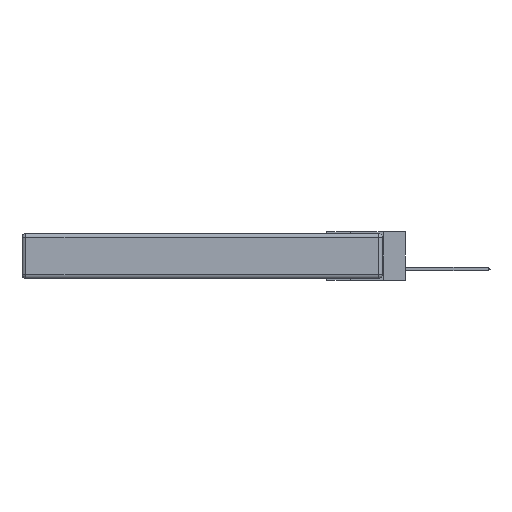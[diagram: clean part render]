
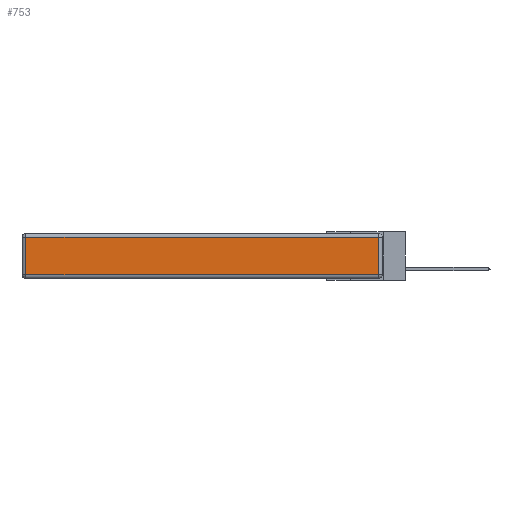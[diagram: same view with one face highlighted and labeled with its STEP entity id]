
A CAD part, left-side view. The second image highlights one B-rep face of the part: STEP entity #753.
In plain terms, the highlighted planar face has unit normal (-1, 0, 0).
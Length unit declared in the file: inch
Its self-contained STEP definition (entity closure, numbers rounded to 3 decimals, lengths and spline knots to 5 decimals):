
#368 = EDGE_LOOP ( 'NONE', ( #6612, #5423, #10526, #2184 ) ) ;
#753 = ADVANCED_FACE ( 'NONE', ( #3915 ), #14682, .T. ) ;
#966 = VERTEX_POINT ( 'NONE', #8173 ) ;
#1011 = VERTEX_POINT ( 'NONE', #5994 ) ;
#1536 = LINE ( 'NONE', #10041, #2439 ) ;
#1815 = DIRECTION ( 'NONE',  ( 0., 1., 0. ) ) ;
#1923 = CARTESIAN_POINT ( 'NONE',  ( 0., 0., -0.343 ) ) ;
#2184 = ORIENTED_EDGE ( 'NONE', *, *, #7579, .T. ) ;
#2439 = VECTOR ( 'NONE', #11105, 39.37008 ) ;
#2649 = AXIS2_PLACEMENT_3D ( 'NONE', #1923, #10116, #7851 ) ;
#3911 = LINE ( 'NONE', #10611, #14487 ) ;
#3915 = FACE_OUTER_BOUND ( 'NONE', #368, .T. ) ;
#4009 = VERTEX_POINT ( 'NONE', #6606 ) ;
#4756 = VERTEX_POINT ( 'NONE', #5354 ) ;
#5354 = CARTESIAN_POINT ( 'NONE',  ( 0., 2.72, -0.313 ) ) ;
#5423 = ORIENTED_EDGE ( 'NONE', *, *, #12907, .T. ) ;
#5526 = CARTESIAN_POINT ( 'NONE',  ( 0., 2.75, -0.03 ) ) ;
#5942 = VECTOR ( 'NONE', #14216, 39.37008 ) ;
#5994 = CARTESIAN_POINT ( 'NONE',  ( 0., 2.72, -0.03 ) ) ;
#6606 = CARTESIAN_POINT ( 'NONE',  ( 0., 0.03, -0.313 ) ) ;
#6612 = ORIENTED_EDGE ( 'NONE', *, *, #12683, .T. ) ;
#7579 = EDGE_CURVE ( 'NONE', #1011, #4756, #9051, .T. ) ;
#7851 = DIRECTION ( 'NONE',  ( 0., 0., 1. ) ) ;
#8173 = CARTESIAN_POINT ( 'NONE',  ( 0., 0.03, -0.03 ) ) ;
#9051 = LINE ( 'NONE', #11870, #5942 ) ;
#9720 = LINE ( 'NONE', #5526, #11170 ) ;
#10041 = CARTESIAN_POINT ( 'NONE',  ( 0., 0., -0.313 ) ) ;
#10116 = DIRECTION ( 'NONE',  ( -1., 0., 0. ) ) ;
#10512 = DIRECTION ( 'NONE',  ( 0., 0., 1. ) ) ;
#10526 = ORIENTED_EDGE ( 'NONE', *, *, #14664, .T. ) ;
#10611 = CARTESIAN_POINT ( 'NONE',  ( 0., 0.03, -0.343 ) ) ;
#11105 = DIRECTION ( 'NONE',  ( 0., -1., 0. ) ) ;
#11170 = VECTOR ( 'NONE', #1815, 39.37008 ) ;
#11870 = CARTESIAN_POINT ( 'NONE',  ( 0., 2.72, -0.343 ) ) ;
#12683 = EDGE_CURVE ( 'NONE', #4756, #4009, #1536, .T. ) ;
#12907 = EDGE_CURVE ( 'NONE', #4009, #966, #3911, .T. ) ;
#14216 = DIRECTION ( 'NONE',  ( 0., 0., -1. ) ) ;
#14487 = VECTOR ( 'NONE', #10512, 39.37008 ) ;
#14664 = EDGE_CURVE ( 'NONE', #966, #1011, #9720, .T. ) ;
#14682 = PLANE ( 'NONE',  #2649 ) ;
